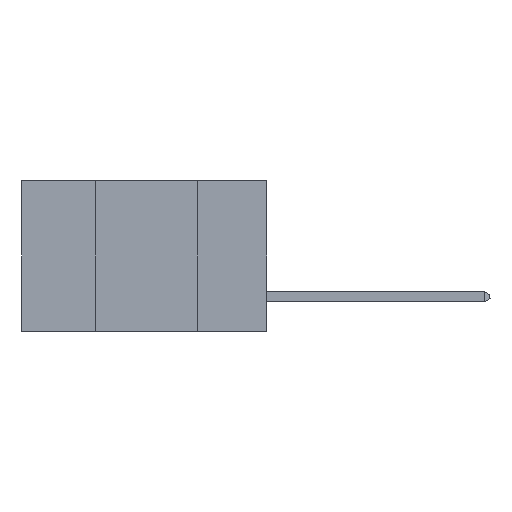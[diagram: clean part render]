
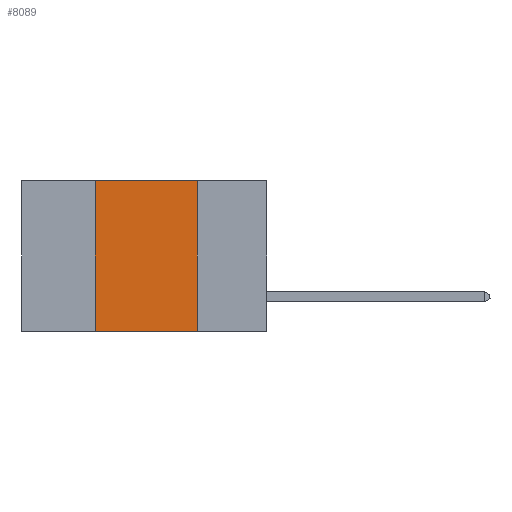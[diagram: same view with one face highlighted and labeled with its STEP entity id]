
A CAD part, left-side view. The second image highlights one B-rep face of the part: STEP entity #8089.
In plain terms, the highlighted planar face has unit normal (-1, 0, 0).
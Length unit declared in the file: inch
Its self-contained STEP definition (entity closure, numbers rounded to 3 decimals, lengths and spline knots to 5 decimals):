
#455 = FACE_OUTER_BOUND ( 'NONE', #18681, .T. ) ;
#902 = EDGE_CURVE ( 'NONE', #17639, #992, #18630, .T. ) ;
#992 = VERTEX_POINT ( 'NONE', #15334 ) ;
#1263 = LINE ( 'NONE', #17221, #12471 ) ;
#2668 = CARTESIAN_POINT ( 'NONE',  ( 0., 0.17, 0. ) ) ;
#2741 = ORIENTED_EDGE ( 'NONE', *, *, #4815, .F. ) ;
#4815 = EDGE_CURVE ( 'NONE', #19066, #9738, #1263, .T. ) ;
#5224 = PLANE ( 'NONE',  #11326 ) ;
#5435 = EDGE_CURVE ( 'NONE', #992, #19066, #14086, .T. ) ;
#5851 = EDGE_CURVE ( 'NONE', #17639, #9738, #15491, .T. ) ;
#6193 = CARTESIAN_POINT ( 'NONE',  ( 0., 0.17, -0.37 ) ) ;
#6324 = ORIENTED_EDGE ( 'NONE', *, *, #5851, .T. ) ;
#6653 = CARTESIAN_POINT ( 'NONE',  ( 0., 0.6, 0. ) ) ;
#7001 = DIRECTION ( 'NONE',  ( 0., -1., 0. ) ) ;
#8089 = ADVANCED_FACE ( 'NONE', ( #455 ), #5224, .F. ) ;
#8607 = DIRECTION ( 'NONE',  ( 0., -1., 0. ) ) ;
#9659 = DIRECTION ( 'NONE',  ( 0., 0., -1. ) ) ;
#9738 = VERTEX_POINT ( 'NONE', #6193 ) ;
#9925 = VECTOR ( 'NONE', #18066, 39.37008 ) ;
#10106 = CARTESIAN_POINT ( 'NONE',  ( 0., 0.6, 0. ) ) ;
#11049 = CARTESIAN_POINT ( 'NONE',  ( 0., 0.42, -0.37 ) ) ;
#11196 = DIRECTION ( 'NONE',  ( 1., 0., 0. ) ) ;
#11326 = AXIS2_PLACEMENT_3D ( 'NONE', #6653, #11196, #9659 ) ;
#12425 = VECTOR ( 'NONE', #8607, 39.37008 ) ;
#12471 = VECTOR ( 'NONE', #18040, 39.37008 ) ;
#14086 = LINE ( 'NONE', #10106, #17589 ) ;
#14142 = ORIENTED_EDGE ( 'NONE', *, *, #5435, .F. ) ;
#15334 = CARTESIAN_POINT ( 'NONE',  ( 0., 0.42, 0. ) ) ;
#15491 = LINE ( 'NONE', #17512, #12425 ) ;
#17221 = CARTESIAN_POINT ( 'NONE',  ( 0., 0.17, 0. ) ) ;
#17512 = CARTESIAN_POINT ( 'NONE',  ( 0., 0.6, -0.37 ) ) ;
#17589 = VECTOR ( 'NONE', #7001, 39.37008 ) ;
#17639 = VERTEX_POINT ( 'NONE', #11049 ) ;
#17965 = ORIENTED_EDGE ( 'NONE', *, *, #902, .F. ) ;
#17993 = CARTESIAN_POINT ( 'NONE',  ( 0., 0.42, 0. ) ) ;
#18040 = DIRECTION ( 'NONE',  ( 0., 0., -1. ) ) ;
#18066 = DIRECTION ( 'NONE',  ( 0., 0., 1. ) ) ;
#18630 = LINE ( 'NONE', #17993, #9925 ) ;
#18681 = EDGE_LOOP ( 'NONE', ( #2741, #14142, #17965, #6324 ) ) ;
#19066 = VERTEX_POINT ( 'NONE', #2668 ) ;
